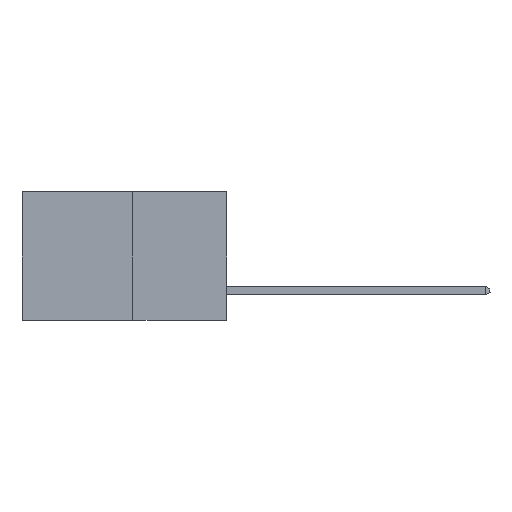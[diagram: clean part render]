
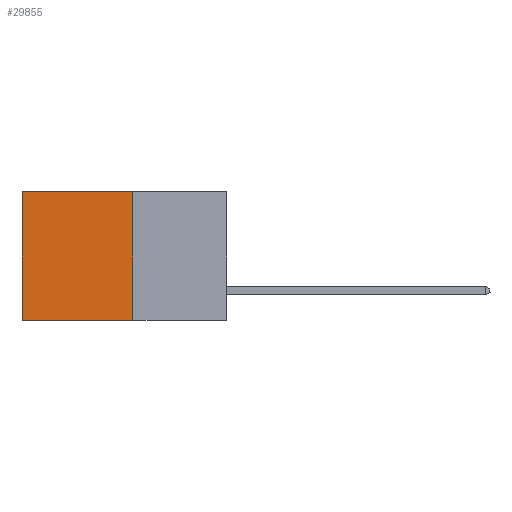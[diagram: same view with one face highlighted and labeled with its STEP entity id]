
A CAD part, left-side view. The second image highlights one B-rep face of the part: STEP entity #29855.
In plain terms, the highlighted planar face has unit normal (-1, 0, 0).
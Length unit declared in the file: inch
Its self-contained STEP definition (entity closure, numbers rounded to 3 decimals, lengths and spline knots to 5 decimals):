
#704 = DIRECTION ( 'NONE',  ( 0., 0., -1. ) ) ;
#1738 = ORIENTED_EDGE ( 'NONE', *, *, #11939, .F. ) ;
#1985 = ORIENTED_EDGE ( 'NONE', *, *, #29388, .T. ) ;
#3326 = ORIENTED_EDGE ( 'NONE', *, *, #12108, .F. ) ;
#4003 = CARTESIAN_POINT ( 'NONE',  ( 0.277, 0.59, -0.37 ) ) ;
#4103 = LINE ( 'NONE', #29837, #16214 ) ;
#4918 = LINE ( 'NONE', #30227, #30756 ) ;
#5001 = CARTESIAN_POINT ( 'NONE',  ( 0.277, 0.27, -0.37 ) ) ;
#6147 = VECTOR ( 'NONE', #27779, 39.37008 ) ;
#7328 = PLANE ( 'NONE',  #29268 ) ;
#7433 = DIRECTION ( 'NONE',  ( 0., 0., -1. ) ) ;
#8275 = VERTEX_POINT ( 'NONE', #28371 ) ;
#11762 = FACE_OUTER_BOUND ( 'NONE', #19118, .T. ) ;
#11939 = EDGE_CURVE ( 'NONE', #28256, #8275, #23947, .T. ) ;
#12108 = EDGE_CURVE ( 'NONE', #8275, #18989, #4918, .T. ) ;
#15613 = CARTESIAN_POINT ( 'NONE',  ( 0.277, 0.27, 0. ) ) ;
#15631 = DIRECTION ( 'NONE',  ( 0., 1., 0. ) ) ;
#16214 = VECTOR ( 'NONE', #704, 39.37008 ) ;
#18989 = VERTEX_POINT ( 'NONE', #4003 ) ;
#19118 = EDGE_LOOP ( 'NONE', ( #31019, #3326, #1738, #1985 ) ) ;
#21015 = CARTESIAN_POINT ( 'NONE',  ( 0.277, 0.59, 0. ) ) ;
#22051 = DIRECTION ( 'NONE',  ( 1., 0., 0. ) ) ;
#22914 = CARTESIAN_POINT ( 'NONE',  ( 0.277, 0.27, 0. ) ) ;
#23947 = LINE ( 'NONE', #29483, #29648 ) ;
#24706 = DIRECTION ( 'NONE',  ( 0., 0., -1. ) ) ;
#25404 = EDGE_CURVE ( 'NONE', #30826, #18989, #4103, .T. ) ;
#27779 = DIRECTION ( 'NONE',  ( 0., 1., 0. ) ) ;
#28256 = VERTEX_POINT ( 'NONE', #22914 ) ;
#28371 = CARTESIAN_POINT ( 'NONE',  ( 0.277, 0.27, -0.37 ) ) ;
#29268 = AXIS2_PLACEMENT_3D ( 'NONE', #5001, #22051, #7433 ) ;
#29388 = EDGE_CURVE ( 'NONE', #28256, #30826, #31206, .T. ) ;
#29483 = CARTESIAN_POINT ( 'NONE',  ( 0.277, 0.27, -0.37 ) ) ;
#29648 = VECTOR ( 'NONE', #24706, 39.37008 ) ;
#29837 = CARTESIAN_POINT ( 'NONE',  ( 0.277, 0.59, -0.37 ) ) ;
#29855 = ADVANCED_FACE ( 'NONE', ( #11762 ), #7328, .F. ) ;
#30227 = CARTESIAN_POINT ( 'NONE',  ( 0.277, 0.27, -0.37 ) ) ;
#30756 = VECTOR ( 'NONE', #15631, 39.37008 ) ;
#30826 = VERTEX_POINT ( 'NONE', #21015 ) ;
#31019 = ORIENTED_EDGE ( 'NONE', *, *, #25404, .T. ) ;
#31206 = LINE ( 'NONE', #15613, #6147 ) ;
